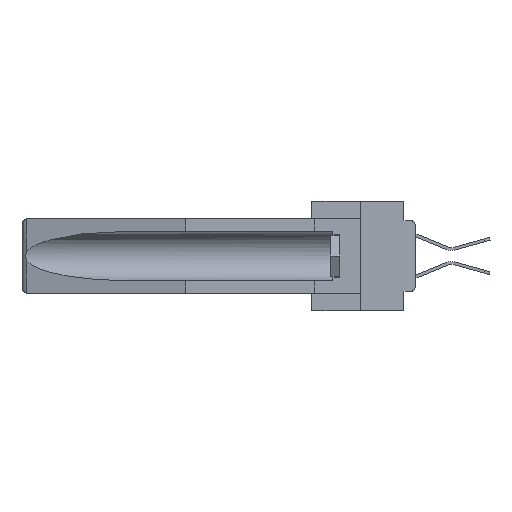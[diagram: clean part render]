
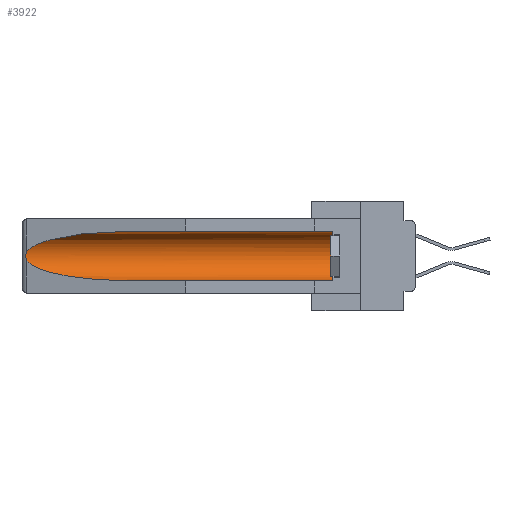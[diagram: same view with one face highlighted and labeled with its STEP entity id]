
A CAD part, left-side view. The second image highlights one B-rep face of the part: STEP entity #3922.
In plain terms, the highlighted cylindrical face has radius 2.857 mm (diameter 5.715 mm), a partial arc.
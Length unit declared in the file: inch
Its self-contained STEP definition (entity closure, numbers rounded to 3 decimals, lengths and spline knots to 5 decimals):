
#488 = CARTESIAN_POINT ( 'NONE',  ( 0.155, 0.126, -0.284 ) ) ;
#1429 = CIRCLE ( 'NONE', #19687, 0.1125 ) ;
#2046 = VERTEX_POINT ( 'NONE', #21696 ) ;
#2527 = AXIS2_PLACEMENT_3D ( 'NONE', #21487, #26448, #7291 ) ;
#2559 = CARTESIAN_POINT ( 'NONE',  ( 0.25451, 1.48313, -0.24835 ) ) ;
#2761 = CARTESIAN_POINT ( 'NONE',  ( 0.26537, 1.52718, -0.14972 ) ) ;
#3295 = ORIENTED_EDGE ( 'NONE', *, *, #9284, .T. ) ;
#3331 = VERTEX_POINT ( 'NONE', #488 ) ;
#3922 = ADVANCED_FACE ( 'NONE', ( #29994 ), #19957, .F. ) ;
#4905 = CARTESIAN_POINT ( 'NONE',  ( 0.26537, 1.52718, -0.19328 ) ) ;
#5477 =( BOUNDED_CURVE ( )  B_SPLINE_CURVE ( 3, ( #5917, #22469, #22664, #8473 ),
 .UNSPECIFIED., .F., .F. ) 
 B_SPLINE_CURVE_WITH_KNOTS ( ( 4, 4 ),
 ( 4.71239, 6.08839 ),
 .UNSPECIFIED. ) 
 CURVE ( )  GEOMETRIC_REPRESENTATION_ITEM ( )  RATIONAL_B_SPLINE_CURVE ( ( 1., 0.848, 0.848, 1. ) ) 
 REPRESENTATION_ITEM ( '' )  );
#5867 = CARTESIAN_POINT ( 'NONE',  ( 0.26537, 1.52718, -0.19328 ) ) ;
#5917 = CARTESIAN_POINT ( 'NONE',  ( 0.155, 1.07973, -0.059 ) ) ;
#6381 = VERTEX_POINT ( 'NONE', #25011 ) ;
#6607 = EDGE_CURVE ( 'NONE', #7822, #13786, #12704, .T. ) ;
#7291 = DIRECTION ( 'NONE',  ( 0., 0., 1. ) ) ;
#7822 = VERTEX_POINT ( 'NONE', #2761 ) ;
#7969 = EDGE_CURVE ( 'NONE', #6381, #2046, #20085, .T. ) ;
#8228 = DIRECTION ( 'NONE',  ( 0., 1., 0. ) ) ;
#8473 = CARTESIAN_POINT ( 'NONE',  ( 0.26537, 1.52718, -0.14972 ) ) ;
#9284 = EDGE_CURVE ( 'NONE', #2046, #7822, #5477, .T. ) ;
#9442 = CARTESIAN_POINT ( 'NONE',  ( 0.2675, 1.53308, -0.16763 ) ) ;
#9583 = CARTESIAN_POINT ( 'NONE',  ( 0.155, -0.30754, -0.284 ) ) ;
#9649 = CARTESIAN_POINT ( 'NONE',  ( 0.2675, 1.53308, -0.17534 ) ) ;
#10696 = EDGE_CURVE ( 'NONE', #3331, #6381, #1429, .T. ) ;
#11053 = ORIENTED_EDGE ( 'NONE', *, *, #7969, .T. ) ;
#11190 = CARTESIAN_POINT ( 'NONE',  ( 0.155, 1.07973, -0.284 ) ) ;
#11299 = VECTOR ( 'NONE', #14313, 39.37008 ) ;
#12006 = CARTESIAN_POINT ( 'NONE',  ( 0.26537, 1.52718, -0.14972 ) ) ;
#12108 = CARTESIAN_POINT ( 'NONE',  ( 0.2673, 1.53269, -0.17917 ) ) ;
#12473 = EDGE_CURVE ( 'NONE', #13786, #17623, #15129, .T. ) ;
#12481 = EDGE_CURVE ( 'NONE', #3331, #17623, #26510, .T. ) ;
#12704 = B_SPLINE_CURVE_WITH_KNOTS ( 'NONE', 3,
 ( #12006, #25929, #28622, #19078, #9442, #9649, #12108, #23644, #18776, #4905 ),
 .UNSPECIFIED., .F., .F.,
 ( 4, 2, 2, 2, 4 ),
 ( 0., 0.00029, 0.00058, 0.00087, 0.00117 ),
 .UNSPECIFIED. ) ;
#13786 = VERTEX_POINT ( 'NONE', #5867 ) ;
#14313 = DIRECTION ( 'NONE',  ( 0., 1., 0. ) ) ;
#14510 = CARTESIAN_POINT ( 'NONE',  ( 0.26537, 1.52718, -0.19328 ) ) ;
#15129 =( BOUNDED_CURVE ( )  B_SPLINE_CURVE ( 3, ( #14510, #2559, #25963, #28553 ),
 .UNSPECIFIED., .F., .F. ) 
 B_SPLINE_CURVE_WITH_KNOTS ( ( 4, 4 ),
 ( 0.1948, 1.5708 ),
 .UNSPECIFIED. ) 
 CURVE ( )  GEOMETRIC_REPRESENTATION_ITEM ( )  RATIONAL_B_SPLINE_CURVE ( ( 1., 0.848, 0.848, 1. ) ) 
 REPRESENTATION_ITEM ( '' )  );
#15422 = ORIENTED_EDGE ( 'NONE', *, *, #12481, .F. ) ;
#15460 = CARTESIAN_POINT ( 'NONE',  ( 0.155, -0.30754, -0.059 ) ) ;
#15842 = ORIENTED_EDGE ( 'NONE', *, *, #6607, .T. ) ;
#16136 = DIRECTION ( 'NONE',  ( 0., -1., 0. ) ) ;
#17623 = VERTEX_POINT ( 'NONE', #11190 ) ;
#18306 = ORIENTED_EDGE ( 'NONE', *, *, #10696, .T. ) ;
#18776 = CARTESIAN_POINT ( 'NONE',  ( 0.26597, 1.5296, -0.19026 ) ) ;
#19078 = CARTESIAN_POINT ( 'NONE',  ( 0.2673, 1.5327, -0.16383 ) ) ;
#19687 = AXIS2_PLACEMENT_3D ( 'NONE', #23192, #16136, #26007 ) ;
#19957 = CYLINDRICAL_SURFACE ( 'NONE', #2527, 0.1125 ) ;
#20085 = LINE ( 'NONE', #15460, #28620 ) ;
#21487 = CARTESIAN_POINT ( 'NONE',  ( 0.155, -0.30754, -0.1715 ) ) ;
#21696 = CARTESIAN_POINT ( 'NONE',  ( 0.155, 1.07973, -0.059 ) ) ;
#22469 = CARTESIAN_POINT ( 'NONE',  ( 0.21114, 1.30732, -0.059 ) ) ;
#22664 = CARTESIAN_POINT ( 'NONE',  ( 0.25451, 1.48313, -0.09465 ) ) ;
#23192 = CARTESIAN_POINT ( 'NONE',  ( 0.155, 0.126, -0.1715 ) ) ;
#23644 = CARTESIAN_POINT ( 'NONE',  ( 0.26655, 1.53094, -0.18657 ) ) ;
#23814 = EDGE_LOOP ( 'NONE', ( #3295, #15842, #27419, #15422, #18306, #11053 ) ) ;
#25011 = CARTESIAN_POINT ( 'NONE',  ( 0.155, 0.126, -0.059 ) ) ;
#25929 = CARTESIAN_POINT ( 'NONE',  ( 0.26597, 1.52961, -0.15275 ) ) ;
#25963 = CARTESIAN_POINT ( 'NONE',  ( 0.21114, 1.30732, -0.284 ) ) ;
#26007 = DIRECTION ( 'NONE',  ( 0., 0., 1. ) ) ;
#26448 = DIRECTION ( 'NONE',  ( 0., 1., 0. ) ) ;
#26510 = LINE ( 'NONE', #9583, #11299 ) ;
#27419 = ORIENTED_EDGE ( 'NONE', *, *, #12473, .T. ) ;
#28553 = CARTESIAN_POINT ( 'NONE',  ( 0.155, 1.07973, -0.284 ) ) ;
#28620 = VECTOR ( 'NONE', #8228, 39.37008 ) ;
#28622 = CARTESIAN_POINT ( 'NONE',  ( 0.26654, 1.53092, -0.15636 ) ) ;
#29994 = FACE_OUTER_BOUND ( 'NONE', #23814, .T. ) ;
